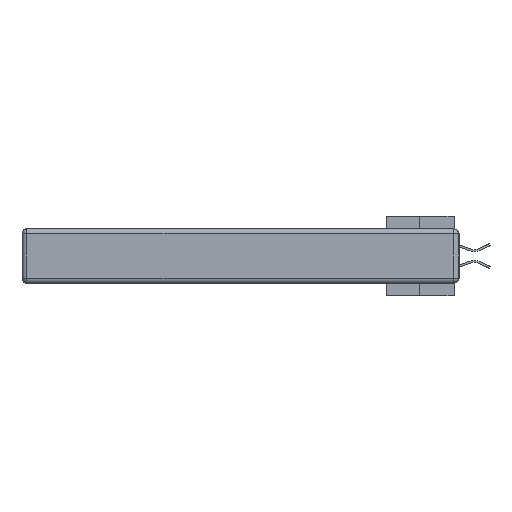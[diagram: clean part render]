
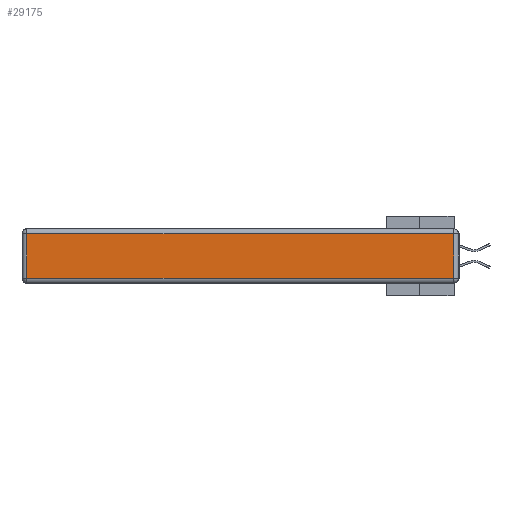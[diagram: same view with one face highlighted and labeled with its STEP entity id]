
A CAD part, left-side view. The second image highlights one B-rep face of the part: STEP entity #29175.
In plain terms, the highlighted planar face has unit normal (-1, 0, 0).
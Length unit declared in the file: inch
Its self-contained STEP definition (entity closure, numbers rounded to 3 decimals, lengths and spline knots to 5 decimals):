
#698 = DIRECTION ( 'NONE',  ( 0., 1., 0. ) ) ;
#2397 = VECTOR ( 'NONE', #698, 39.37008 ) ;
#2724 = VERTEX_POINT ( 'NONE', #14801 ) ;
#4027 = ORIENTED_EDGE ( 'NONE', *, *, #33408, .T. ) ;
#6647 = CARTESIAN_POINT ( 'NONE',  ( 0., 2.72, -0.03 ) ) ;
#6698 = VECTOR ( 'NONE', #45878, 39.37008 ) ;
#8319 = CARTESIAN_POINT ( 'NONE',  ( 0., 0.03, -0.343 ) ) ;
#9122 = DIRECTION ( 'NONE',  ( 0., -1., 0. ) ) ;
#9269 = ORIENTED_EDGE ( 'NONE', *, *, #28850, .T. ) ;
#10251 = AXIS2_PLACEMENT_3D ( 'NONE', #14373, #25564, #33493 ) ;
#10545 = LINE ( 'NONE', #19092, #21692 ) ;
#11409 = CARTESIAN_POINT ( 'NONE',  ( 0., 2.72, -0.343 ) ) ;
#11834 = VERTEX_POINT ( 'NONE', #31390 ) ;
#12091 = ORIENTED_EDGE ( 'NONE', *, *, #30371, .T. ) ;
#14289 = CARTESIAN_POINT ( 'NONE',  ( 0., 0.03, -0.313 ) ) ;
#14373 = CARTESIAN_POINT ( 'NONE',  ( 0., 0., -0.343 ) ) ;
#14801 = CARTESIAN_POINT ( 'NONE',  ( 0., 0.03, -0.03 ) ) ;
#17540 = EDGE_CURVE ( 'NONE', #41240, #2724, #42996, .T. ) ;
#19092 = CARTESIAN_POINT ( 'NONE',  ( 0., 0., -0.313 ) ) ;
#21692 = VECTOR ( 'NONE', #9122, 39.37008 ) ;
#23306 = CARTESIAN_POINT ( 'NONE',  ( 0., 2.75, -0.03 ) ) ;
#24676 = FACE_OUTER_BOUND ( 'NONE', #34132, .T. ) ;
#25564 = DIRECTION ( 'NONE',  ( -1., 0., 0. ) ) ;
#28850 = EDGE_CURVE ( 'NONE', #2724, #46113, #41040, .T. ) ;
#29175 = ADVANCED_FACE ( 'NONE', ( #24676 ), #37088, .T. ) ;
#30371 = EDGE_CURVE ( 'NONE', #11834, #41240, #10545, .T. ) ;
#30575 = ORIENTED_EDGE ( 'NONE', *, *, #17540, .T. ) ;
#31390 = CARTESIAN_POINT ( 'NONE',  ( 0., 2.72, -0.313 ) ) ;
#32071 = VECTOR ( 'NONE', #33962, 39.37008 ) ;
#33408 = EDGE_CURVE ( 'NONE', #46113, #11834, #34950, .T. ) ;
#33493 = DIRECTION ( 'NONE',  ( 0., 0., 1. ) ) ;
#33962 = DIRECTION ( 'NONE',  ( 0., 0., -1. ) ) ;
#34132 = EDGE_LOOP ( 'NONE', ( #12091, #30575, #9269, #4027 ) ) ;
#34950 = LINE ( 'NONE', #11409, #32071 ) ;
#37088 = PLANE ( 'NONE',  #10251 ) ;
#41040 = LINE ( 'NONE', #23306, #2397 ) ;
#41240 = VERTEX_POINT ( 'NONE', #14289 ) ;
#42996 = LINE ( 'NONE', #8319, #6698 ) ;
#45878 = DIRECTION ( 'NONE',  ( 0., 0., 1. ) ) ;
#46113 = VERTEX_POINT ( 'NONE', #6647 ) ;
